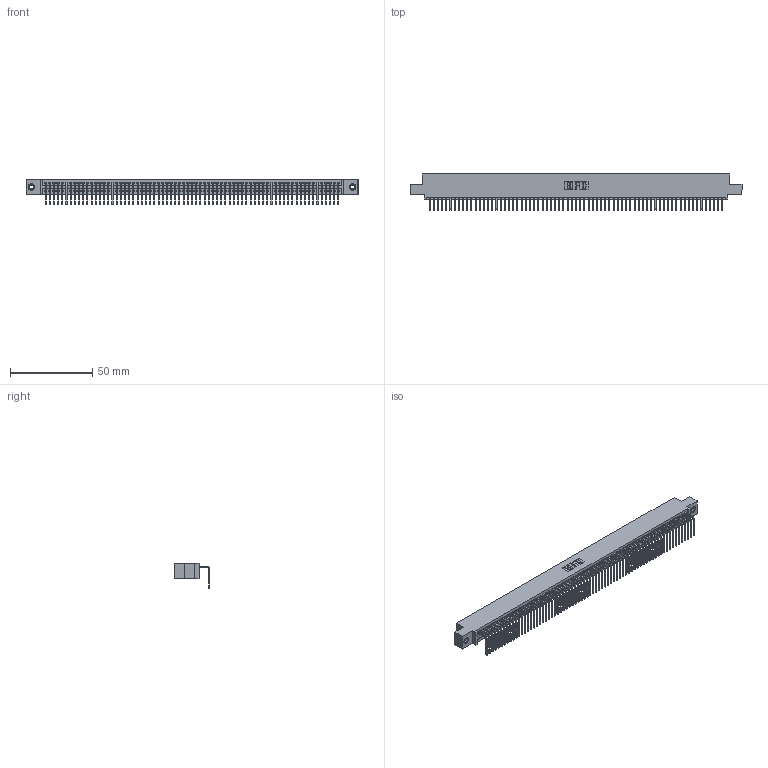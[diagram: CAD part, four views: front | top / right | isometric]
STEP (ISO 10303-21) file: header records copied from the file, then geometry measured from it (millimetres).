
FILE_DESCRIPTION (( 'STEP AP203' ), '1' );
FILE_NAME ('345-071-558-408.STEP', '2018-10-01T16:27:38', ( '' ), ( '' ), 'SwSTEP 2.0', 'SolidWorks 2016', '' );
FILE_SCHEMA (( 'CONFIG_CONTROL_DESIGN' ));
Length unit declared in the file: inch
Products named in the file (4): 345-292-001_558 Tail - 2; 345 Part_0.110 Offset - 0.156 Dia-TI; 345-071-558-408; 345-250-001_345-250-003-102
Assembly tree (74 placements, depth 2):
  345-071-558-408
    345 Part_0.110 Offset - 0.156 Dia-TI
    345-292-001_558 Tail - 2  x71
    345-250-001_345-250-003-102  x2
Bounding box: 201.55 x 21.83 x 15.37 mm (x, y, z)
Volume: 19537.6 mm3; surface area: 27848.8 mm2
Topology: 74 solids, 74 shells, 4450 faces, 13411 edges, 8838 vertices
Faces by surface type: plane 3098, cylinder 1336, cone 12, torus 4
Entity records: 50934 total; most frequent: CARTESIAN_POINT 8804, ORIENTED_EDGE 8802, DIRECTION 7673, EDGE_CURVE 4401, VECTOR 3965, LINE 3965, VERTEX_POINT 2928, AXIS2_PLACEMENT_3D 1854
